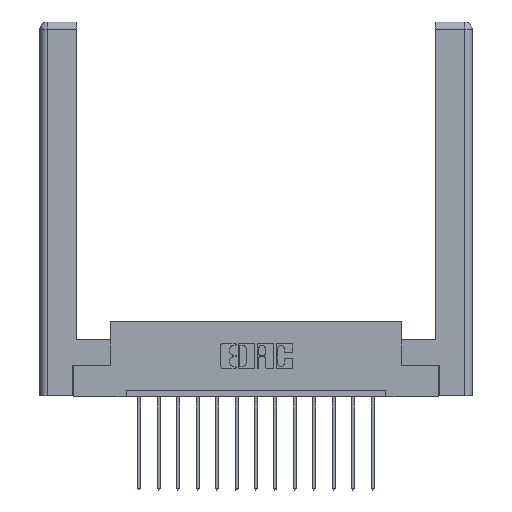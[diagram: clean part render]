
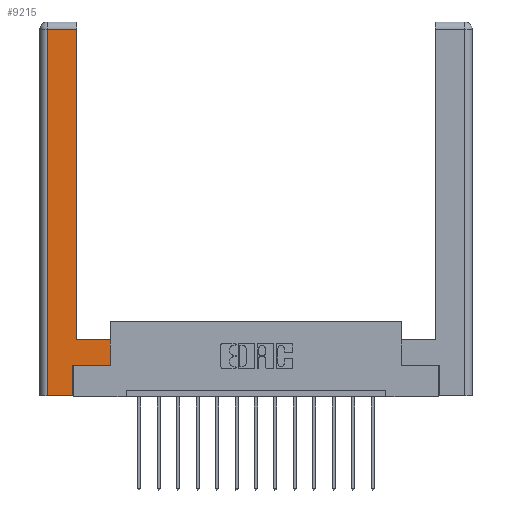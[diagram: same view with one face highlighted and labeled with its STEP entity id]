
A CAD part, top view. The second image highlights one B-rep face of the part: STEP entity #9215.
In plain terms, the highlighted planar face has unit normal (0, 0, 1).
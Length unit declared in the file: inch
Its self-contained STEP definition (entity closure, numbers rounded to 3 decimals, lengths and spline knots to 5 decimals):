
#306 = DIRECTION ( 'NONE',  ( 1., 0., 0. ) ) ;
#522 = VERTEX_POINT ( 'NONE', #12993 ) ;
#845 = CARTESIAN_POINT ( 'NONE',  ( 0.0615, 0., 0. ) ) ;
#1175 = CARTESIAN_POINT ( 'NONE',  ( 0.565, 0.45, 0. ) ) ;
#1361 = CARTESIAN_POINT ( 'NONE',  ( 0.295, 0.45, 0. ) ) ;
#1365 = VECTOR ( 'NONE', #14441, 39.37008 ) ;
#1411 = CARTESIAN_POINT ( 'NONE',  ( 0.0615, 2.94, 0. ) ) ;
#1464 = DIRECTION ( 'NONE',  ( -1., 0., 0. ) ) ;
#1771 = CARTESIAN_POINT ( 'NONE',  ( 0.265, 0.245, 0. ) ) ;
#1870 = DIRECTION ( 'NONE',  ( -1., 0., 0. ) ) ;
#1973 = EDGE_CURVE ( 'NONE', #5644, #3499, #6912, .T. ) ;
#2844 = CARTESIAN_POINT ( 'NONE',  ( 0.265, 0., 0. ) ) ;
#2920 = LINE ( 'NONE', #12484, #4463 ) ;
#3048 = EDGE_CURVE ( 'NONE', #15349, #6586, #5906, .T. ) ;
#3253 = VECTOR ( 'NONE', #1464, 39.37008 ) ;
#3304 = CARTESIAN_POINT ( 'NONE',  ( 0.265, 0., 0. ) ) ;
#3499 = VERTEX_POINT ( 'NONE', #12854 ) ;
#3823 = AXIS2_PLACEMENT_3D ( 'NONE', #8058, #9493, #1870 ) ;
#4268 = ORIENTED_EDGE ( 'NONE', *, *, #5836, .T. ) ;
#4271 = ORIENTED_EDGE ( 'NONE', *, *, #11701, .T. ) ;
#4441 = LINE ( 'NONE', #2844, #9705 ) ;
#4454 = PLANE ( 'NONE',  #3823 ) ;
#4463 = VECTOR ( 'NONE', #5049, 39.37008 ) ;
#5049 = DIRECTION ( 'NONE',  ( 0., 1., 0. ) ) ;
#5171 = CARTESIAN_POINT ( 'NONE',  ( 0.0615, 2.94, 0. ) ) ;
#5644 = VERTEX_POINT ( 'NONE', #1175 ) ;
#5806 = DIRECTION ( 'NONE',  ( 0., 1., 0. ) ) ;
#5836 = EDGE_CURVE ( 'NONE', #3499, #15349, #9784, .T. ) ;
#5906 = LINE ( 'NONE', #1411, #15625 ) ;
#6003 = VECTOR ( 'NONE', #8021, 39.37008 ) ;
#6586 = VERTEX_POINT ( 'NONE', #5171 ) ;
#6645 = ORIENTED_EDGE ( 'NONE', *, *, #1973, .T. ) ;
#6912 = LINE ( 'NONE', #1361, #3253 ) ;
#7375 = VERTEX_POINT ( 'NONE', #3304 ) ;
#7548 = EDGE_CURVE ( 'NONE', #7375, #14878, #14395, .T. ) ;
#7753 = ORIENTED_EDGE ( 'NONE', *, *, #12471, .T. ) ;
#7754 = CARTESIAN_POINT ( 'NONE',  ( 0.295, 3., 0. ) ) ;
#7910 = DIRECTION ( 'NONE',  ( 1., 0., 0. ) ) ;
#7980 = EDGE_CURVE ( 'NONE', #10345, #7375, #4441, .T. ) ;
#8021 = DIRECTION ( 'NONE',  ( 0., -1., 0. ) ) ;
#8058 = CARTESIAN_POINT ( 'NONE',  ( 0., 0., 0. ) ) ;
#9005 = EDGE_CURVE ( 'NONE', #522, #5644, #2920, .T. ) ;
#9215 = ADVANCED_FACE ( 'NONE', ( #11457 ), #4454, .F. ) ;
#9493 = DIRECTION ( 'NONE',  ( 0., 0., -1. ) ) ;
#9705 = VECTOR ( 'NONE', #7910, 39.37008 ) ;
#9746 = ORIENTED_EDGE ( 'NONE', *, *, #7548, .T. ) ;
#9784 = LINE ( 'NONE', #7754, #14454 ) ;
#10215 = CARTESIAN_POINT ( 'NONE',  ( 0.565, 0.245, 0. ) ) ;
#10265 = LINE ( 'NONE', #10215, #15538 ) ;
#10345 = VERTEX_POINT ( 'NONE', #845 ) ;
#10555 = ORIENTED_EDGE ( 'NONE', *, *, #9005, .T. ) ;
#11457 = FACE_OUTER_BOUND ( 'NONE', #15775, .T. ) ;
#11539 = ORIENTED_EDGE ( 'NONE', *, *, #7980, .T. ) ;
#11701 = EDGE_CURVE ( 'NONE', #6586, #10345, #14769, .T. ) ;
#12027 = CARTESIAN_POINT ( 'NONE',  ( 0.295, 2.94, 0. ) ) ;
#12471 = EDGE_CURVE ( 'NONE', #14878, #522, #10265, .T. ) ;
#12484 = CARTESIAN_POINT ( 'NONE',  ( 0.565, 0.45, 0. ) ) ;
#12854 = CARTESIAN_POINT ( 'NONE',  ( 0.295, 0.45, 0. ) ) ;
#12993 = CARTESIAN_POINT ( 'NONE',  ( 0.565, 0.245, 0. ) ) ;
#12999 = CARTESIAN_POINT ( 'NONE',  ( 0.0615, 0., 0. ) ) ;
#14395 = LINE ( 'NONE', #15619, #1365 ) ;
#14441 = DIRECTION ( 'NONE',  ( 0., 1., 0. ) ) ;
#14454 = VECTOR ( 'NONE', #5806, 39.37008 ) ;
#14684 = ORIENTED_EDGE ( 'NONE', *, *, #3048, .T. ) ;
#14769 = LINE ( 'NONE', #12999, #6003 ) ;
#14878 = VERTEX_POINT ( 'NONE', #1771 ) ;
#14935 = DIRECTION ( 'NONE',  ( -1., 0., 0. ) ) ;
#15349 = VERTEX_POINT ( 'NONE', #12027 ) ;
#15538 = VECTOR ( 'NONE', #306, 39.37008 ) ;
#15619 = CARTESIAN_POINT ( 'NONE',  ( 0.265, 0.245, 0. ) ) ;
#15625 = VECTOR ( 'NONE', #14935, 39.37008 ) ;
#15775 = EDGE_LOOP ( 'NONE', ( #4268, #14684, #4271, #11539, #9746, #7753, #10555, #6645 ) ) ;
